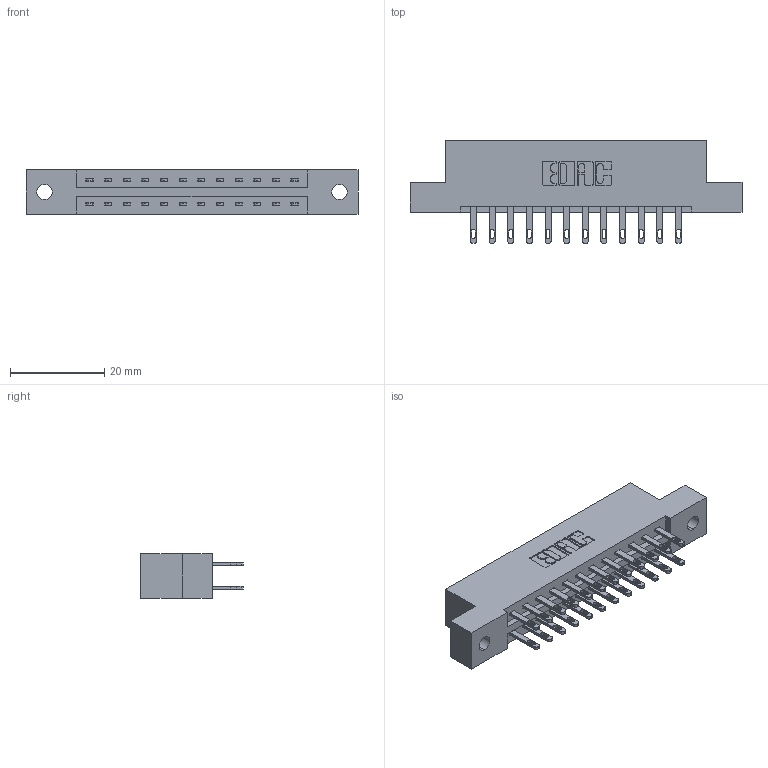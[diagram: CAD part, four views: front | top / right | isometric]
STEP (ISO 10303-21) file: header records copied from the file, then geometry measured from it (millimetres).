
FILE_DESCRIPTION (( 'STEP AP203' ), '1' );
FILE_NAME ('337-024-500-202.STEP', '2019-10-08T15:08:12', ( '' ), ( '' ), 'SwSTEP 2.0', 'SolidWorks 2016', '' );
FILE_SCHEMA (( 'CONFIG_CONTROL_DESIGN' ));
Length unit declared in the file: inch
Products named in the file (3): 345-292-001_345-293-100; 337 Part_Flush Mounting Lugs - 0.128 Dia; 337-024-500-202
Assembly tree (25 placements, depth 2):
  337-024-500-202
    337 Part_Flush Mounting Lugs - 0.128 Dia
    345-292-001_345-293-100  x24
Bounding box: 70.56 x 21.85 x 9.4 mm (x, y, z)
Volume: 7073.6 mm3; surface area: 7698.9 mm2
Topology: 25 solids, 25 shells, 1314 faces, 3983 edges, 2654 vertices
Faces by surface type: plane 838, cylinder 476
Entity records: 13117 total; most frequent: CARTESIAN_POINT 2234, ORIENTED_EDGE 2170, DIRECTION 1957, EDGE_CURVE 1085, VECTOR 953, LINE 953, VERTEX_POINT 722, AXIS2_PLACEMENT_3D 502
